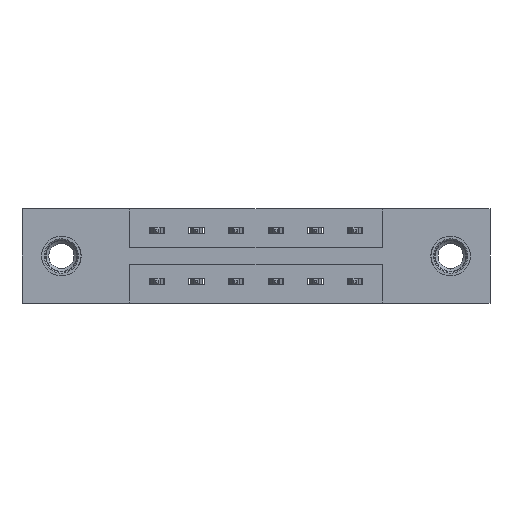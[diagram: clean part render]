
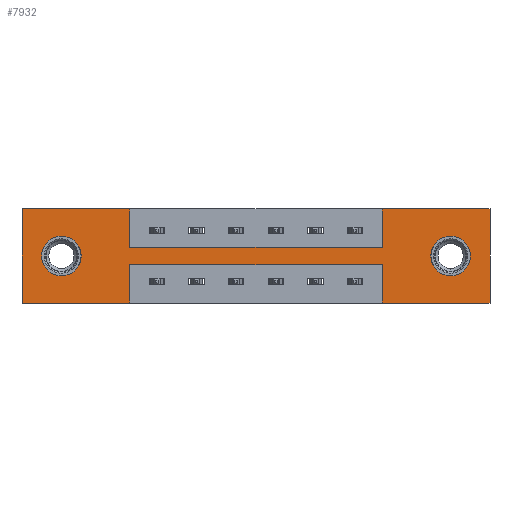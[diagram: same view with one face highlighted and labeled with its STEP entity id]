
A CAD part, front view. The second image highlights one B-rep face of the part: STEP entity #7932.
In plain terms, the highlighted planar face has unit normal (0, -1, 0).
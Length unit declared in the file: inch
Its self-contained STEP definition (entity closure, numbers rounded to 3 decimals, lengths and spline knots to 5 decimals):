
#98 = ORIENTED_EDGE ( 'NONE', *, *, #5654, .F. ) ;
#146 = LINE ( 'NONE', #3922, #4680 ) ;
#551 = CARTESIAN_POINT ( 'NONE',  ( 0., 0., 0. ) ) ;
#713 = CIRCLE ( 'NONE', #3688, 0.078 ) ;
#731 = CARTESIAN_POINT ( 'NONE',  ( 1.842, 0., 0. ) ) ;
#861 = CARTESIAN_POINT ( 'NONE',  ( 0.425, 0., 0. ) ) ;
#1012 = ORIENTED_EDGE ( 'NONE', *, *, #7581, .T. ) ;
#1194 = LINE ( 'NONE', #551, #3133 ) ;
#1213 = VERTEX_POINT ( 'NONE', #8789 ) ;
#1289 = ORIENTED_EDGE ( 'NONE', *, *, #6448, .F. ) ;
#1396 = EDGE_CURVE ( 'NONE', #7364, #2620, #8136, .T. ) ;
#1789 = CIRCLE ( 'NONE', #8405, 0.078 ) ;
#1824 = ORIENTED_EDGE ( 'NONE', *, *, #3577, .F. ) ;
#1911 = VERTEX_POINT ( 'NONE', #8523 ) ;
#1974 = CARTESIAN_POINT ( 'NONE',  ( 1.417, 0., -0.37 ) ) ;
#1994 = CARTESIAN_POINT ( 'NONE',  ( 1.417, 0., -0.22 ) ) ;
#2090 = ORIENTED_EDGE ( 'NONE', *, *, #3763, .F. ) ;
#2149 = EDGE_LOOP ( 'NONE', ( #1289, #7790, #3707, #8039, #1824, #6061, #8297, #10403, #2090, #8562, #98, #2355 ) ) ;
#2272 = DIRECTION ( 'NONE',  ( -1., 0., 0. ) ) ;
#2285 = VERTEX_POINT ( 'NONE', #5771 ) ;
#2350 = VERTEX_POINT ( 'NONE', #4640 ) ;
#2355 = ORIENTED_EDGE ( 'NONE', *, *, #9767, .F. ) ;
#2423 = DIRECTION ( 'NONE',  ( 0., 0., 1. ) ) ;
#2620 = VERTEX_POINT ( 'NONE', #3605 ) ;
#2733 = CARTESIAN_POINT ( 'NONE',  ( 0.155, 0., -0.263 ) ) ;
#2745 = VECTOR ( 'NONE', #4362, 39.37008 ) ;
#2913 = CARTESIAN_POINT ( 'NONE',  ( 0.155, 0., -0.185 ) ) ;
#2992 = CARTESIAN_POINT ( 'NONE',  ( 0.425, 0., -0.37 ) ) ;
#2995 = EDGE_LOOP ( 'NONE', ( #5249, #7511 ) ) ;
#3045 = LINE ( 'NONE', #4519, #7067 ) ;
#3055 = DIRECTION ( 'NONE',  ( 0., 0., 1. ) ) ;
#3133 = VECTOR ( 'NONE', #2423, 39.37008 ) ;
#3156 = VERTEX_POINT ( 'NONE', #4745 ) ;
#3158 = DIRECTION ( 'NONE',  ( 0., 1., 0. ) ) ;
#3220 = ORIENTED_EDGE ( 'NONE', *, *, #10273, .T. ) ;
#3246 = VECTOR ( 'NONE', #8637, 39.37008 ) ;
#3308 = LINE ( 'NONE', #8148, #7327 ) ;
#3572 = CIRCLE ( 'NONE', #6290, 0.078 ) ;
#3577 = EDGE_CURVE ( 'NONE', #2350, #7364, #10335, .T. ) ;
#3605 = CARTESIAN_POINT ( 'NONE',  ( 1.417, 0., -0.37 ) ) ;
#3688 = AXIS2_PLACEMENT_3D ( 'NONE', #8018, #3158, #8850 ) ;
#3703 = DIRECTION ( 'NONE',  ( 0., 0., 1. ) ) ;
#3707 = ORIENTED_EDGE ( 'NONE', *, *, #5304, .F. ) ;
#3763 = EDGE_CURVE ( 'NONE', #8411, #5763, #4430, .T. ) ;
#3777 = EDGE_CURVE ( 'NONE', #9361, #2350, #146, .T. ) ;
#3785 = DIRECTION ( 'NONE',  ( 0., 1., 0. ) ) ;
#3840 = DIRECTION ( 'NONE',  ( 0., 0., -1. ) ) ;
#3892 = DIRECTION ( 'NONE',  ( 0., 1., 0. ) ) ;
#3922 = CARTESIAN_POINT ( 'NONE',  ( 0., 0., 0. ) ) ;
#4044 = AXIS2_PLACEMENT_3D ( 'NONE', #7742, #9385, #4412 ) ;
#4048 = DIRECTION ( 'NONE',  ( 1., 0., 0. ) ) ;
#4089 = VERTEX_POINT ( 'NONE', #6494 ) ;
#4163 = VECTOR ( 'NONE', #3055, 39.37008 ) ;
#4247 = EDGE_CURVE ( 'NONE', #5763, #1213, #6907, .T. ) ;
#4362 = DIRECTION ( 'NONE',  ( -1., 0., 0. ) ) ;
#4412 = DIRECTION ( 'NONE',  ( 0., 0., -1. ) ) ;
#4430 = LINE ( 'NONE', #861, #8608 ) ;
#4519 = CARTESIAN_POINT ( 'NONE',  ( 0., 0., 0. ) ) ;
#4640 = CARTESIAN_POINT ( 'NONE',  ( 1.842, 0., 0. ) ) ;
#4680 = VECTOR ( 'NONE', #4048, 39.37008 ) ;
#4745 = CARTESIAN_POINT ( 'NONE',  ( 1.687, 0., -0.107 ) ) ;
#4766 = EDGE_CURVE ( 'NONE', #1213, #9361, #5278, .T. ) ;
#4882 = LINE ( 'NONE', #2992, #7137 ) ;
#4971 = CARTESIAN_POINT ( 'NONE',  ( 1.842, 0., -0.37 ) ) ;
#5172 = VERTEX_POINT ( 'NONE', #9388 ) ;
#5249 = ORIENTED_EDGE ( 'NONE', *, *, #9120, .T. ) ;
#5278 = LINE ( 'NONE', #6656, #3246 ) ;
#5304 = EDGE_CURVE ( 'NONE', #2620, #6814, #8827, .T. ) ;
#5334 = DIRECTION ( 'NONE',  ( 1., 0., 0. ) ) ;
#5433 = VERTEX_POINT ( 'NONE', #5580 ) ;
#5580 = CARTESIAN_POINT ( 'NONE',  ( 0.425, 0., -0.22 ) ) ;
#5623 = FACE_OUTER_BOUND ( 'NONE', #2149, .T. ) ;
#5654 = EDGE_CURVE ( 'NONE', #2285, #7574, #1194, .T. ) ;
#5763 = VERTEX_POINT ( 'NONE', #9166 ) ;
#5771 = CARTESIAN_POINT ( 'NONE',  ( 0., 0., -0.37 ) ) ;
#5884 = EDGE_CURVE ( 'NONE', #6814, #5433, #9476, .T. ) ;
#5906 = FACE_BOUND ( 'NONE', #2995, .T. ) ;
#5980 = CARTESIAN_POINT ( 'NONE',  ( 0.425, 0., -0.22 ) ) ;
#5984 = VECTOR ( 'NONE', #10528, 39.37008 ) ;
#6061 = ORIENTED_EDGE ( 'NONE', *, *, #3777, .F. ) ;
#6099 = CARTESIAN_POINT ( 'NONE',  ( 0., 0., -0.37 ) ) ;
#6290 = AXIS2_PLACEMENT_3D ( 'NONE', #8802, #3892, #9600 ) ;
#6303 = CARTESIAN_POINT ( 'NONE',  ( 0.425, 0., 0. ) ) ;
#6448 = EDGE_CURVE ( 'NONE', #5433, #1911, #4882, .T. ) ;
#6494 = CARTESIAN_POINT ( 'NONE',  ( 0.155, 0., -0.107 ) ) ;
#6656 = CARTESIAN_POINT ( 'NONE',  ( 1.417, 0., 0. ) ) ;
#6814 = VERTEX_POINT ( 'NONE', #1994 ) ;
#6822 = CARTESIAN_POINT ( 'NONE',  ( 0.425, 0., -0.15 ) ) ;
#6874 = AXIS2_PLACEMENT_3D ( 'NONE', #8693, #3785, #9494 ) ;
#6907 = LINE ( 'NONE', #6822, #8857 ) ;
#7067 = VECTOR ( 'NONE', #5334, 39.37008 ) ;
#7137 = VECTOR ( 'NONE', #10231, 39.37008 ) ;
#7327 = VECTOR ( 'NONE', #8976, 39.37008 ) ;
#7364 = VERTEX_POINT ( 'NONE', #4971 ) ;
#7511 = ORIENTED_EDGE ( 'NONE', *, *, #9455, .T. ) ;
#7574 = VERTEX_POINT ( 'NONE', #9568 ) ;
#7581 = EDGE_CURVE ( 'NONE', #3156, #5172, #3572, .T. ) ;
#7742 = CARTESIAN_POINT ( 'NONE',  ( 0., 0., -0.37 ) ) ;
#7790 = ORIENTED_EDGE ( 'NONE', *, *, #5884, .F. ) ;
#7877 = CIRCLE ( 'NONE', #6874, 0.078 ) ;
#7932 = ADVANCED_FACE ( 'NONE', ( #10029, #5906, #5623 ), #8575, .T. ) ;
#8018 = CARTESIAN_POINT ( 'NONE',  ( 0.155, 0., -0.185 ) ) ;
#8039 = ORIENTED_EDGE ( 'NONE', *, *, #1396, .F. ) ;
#8136 = LINE ( 'NONE', #6099, #9776 ) ;
#8148 = CARTESIAN_POINT ( 'NONE',  ( 0., 0., -0.37 ) ) ;
#8297 = ORIENTED_EDGE ( 'NONE', *, *, #4766, .F. ) ;
#8307 = DIRECTION ( 'NONE',  ( 1., 0., 0. ) ) ;
#8405 = AXIS2_PLACEMENT_3D ( 'NONE', #2913, #8591, #3703 ) ;
#8411 = VERTEX_POINT ( 'NONE', #6303 ) ;
#8523 = CARTESIAN_POINT ( 'NONE',  ( 0.425, 0., -0.37 ) ) ;
#8562 = ORIENTED_EDGE ( 'NONE', *, *, #10287, .F. ) ;
#8575 = PLANE ( 'NONE',  #4044 ) ;
#8591 = DIRECTION ( 'NONE',  ( 0., 1., 0. ) ) ;
#8608 = VECTOR ( 'NONE', #3840, 39.37008 ) ;
#8637 = DIRECTION ( 'NONE',  ( 0., 0., 1. ) ) ;
#8693 = CARTESIAN_POINT ( 'NONE',  ( 1.687, 0., -0.185 ) ) ;
#8789 = CARTESIAN_POINT ( 'NONE',  ( 1.417, 0., -0.15 ) ) ;
#8802 = CARTESIAN_POINT ( 'NONE',  ( 1.687, 0., -0.185 ) ) ;
#8827 = LINE ( 'NONE', #1974, #4163 ) ;
#8850 = DIRECTION ( 'NONE',  ( 0., 0., 1. ) ) ;
#8857 = VECTOR ( 'NONE', #8307, 39.37008 ) ;
#8976 = DIRECTION ( 'NONE',  ( -1., 0., 0. ) ) ;
#9120 = EDGE_CURVE ( 'NONE', #4089, #9325, #713, .T. ) ;
#9166 = CARTESIAN_POINT ( 'NONE',  ( 0.425, 0., -0.15 ) ) ;
#9272 = CARTESIAN_POINT ( 'NONE',  ( 1.417, 0., 0. ) ) ;
#9325 = VERTEX_POINT ( 'NONE', #2733 ) ;
#9361 = VERTEX_POINT ( 'NONE', #9272 ) ;
#9385 = DIRECTION ( 'NONE',  ( 0., -1., 0. ) ) ;
#9388 = CARTESIAN_POINT ( 'NONE',  ( 1.687, 0., -0.263 ) ) ;
#9455 = EDGE_CURVE ( 'NONE', #9325, #4089, #1789, .T. ) ;
#9476 = LINE ( 'NONE', #5980, #2745 ) ;
#9494 = DIRECTION ( 'NONE',  ( 0., 0., -1. ) ) ;
#9568 = CARTESIAN_POINT ( 'NONE',  ( 0., 0., 0. ) ) ;
#9600 = DIRECTION ( 'NONE',  ( 0., 0., -1. ) ) ;
#9767 = EDGE_CURVE ( 'NONE', #1911, #2285, #3308, .T. ) ;
#9776 = VECTOR ( 'NONE', #2272, 39.37008 ) ;
#10029 = FACE_BOUND ( 'NONE', #10450, .T. ) ;
#10231 = DIRECTION ( 'NONE',  ( 0., 0., -1. ) ) ;
#10273 = EDGE_CURVE ( 'NONE', #5172, #3156, #7877, .T. ) ;
#10287 = EDGE_CURVE ( 'NONE', #7574, #8411, #3045, .T. ) ;
#10335 = LINE ( 'NONE', #731, #5984 ) ;
#10403 = ORIENTED_EDGE ( 'NONE', *, *, #4247, .F. ) ;
#10450 = EDGE_LOOP ( 'NONE', ( #1012, #3220 ) ) ;
#10528 = DIRECTION ( 'NONE',  ( 0., 0., -1. ) ) ;
